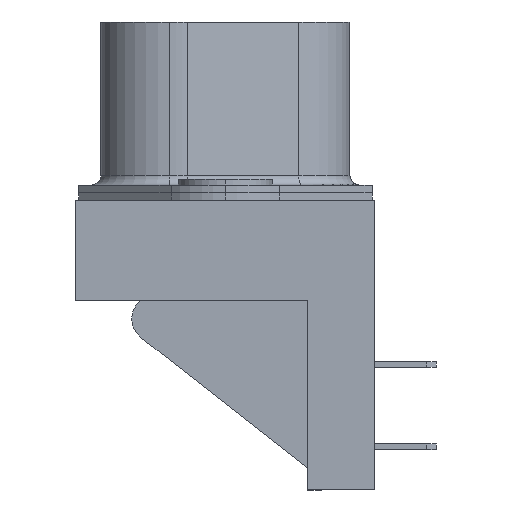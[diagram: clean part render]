
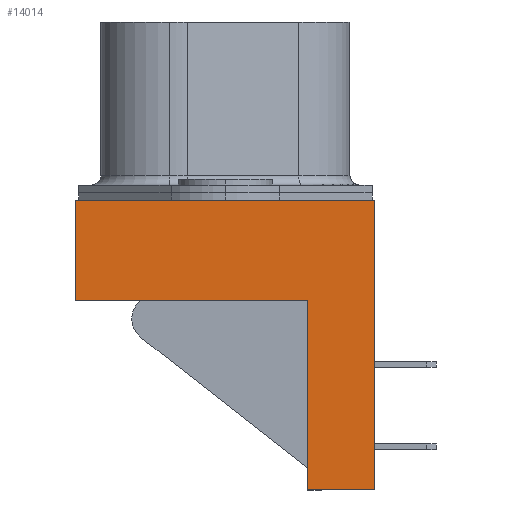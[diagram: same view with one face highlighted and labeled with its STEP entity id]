
A CAD part, left-side view. The second image highlights one B-rep face of the part: STEP entity #14014.
In plain terms, the highlighted planar face has unit normal (-1, 0, 0).
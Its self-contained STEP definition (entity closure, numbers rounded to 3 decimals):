
#9369 = VECTOR ( 'NONE', #12311, 1000. ) ;
#9684 = VECTOR ( 'NONE', #60644, 1000. ) ;
#11759 = AXIS2_PLACEMENT_3D ( 'NONE', #77047, #102448, #144937 ) ;
#12311 = DIRECTION ( 'NONE',  ( 0., 0., 1. ) ) ;
#14014 = ADVANCED_FACE ( 'NONE', ( #63472 ), #129609, .T. ) ;
#18101 = CARTESIAN_POINT ( 'NONE',  ( -4.125, 7.8, -5.2 ) ) ;
#22136 = DIRECTION ( 'NONE',  ( 0., -1., 0. ) ) ;
#24438 = VERTEX_POINT ( 'NONE', #119259 ) ;
#33593 = EDGE_CURVE ( 'NONE', #167851, #145563, #58864, .T. ) ;
#37057 = LINE ( 'NONE', #165261, #9369 ) ;
#38082 = LINE ( 'NONE', #151143, #132666 ) ;
#38355 = EDGE_CURVE ( 'NONE', #89803, #167851, #37057, .T. ) ;
#39267 = EDGE_LOOP ( 'NONE', ( #99872, #169555, #94851, #153107, #139628, #147882 ) ) ;
#40729 = DIRECTION ( 'NONE',  ( 0., 0., 1. ) ) ;
#41414 = LINE ( 'NONE', #83108, #78340 ) ;
#44869 = DIRECTION ( 'NONE',  ( 0., -1., 0. ) ) ;
#58864 = LINE ( 'NONE', #18101, #9684 ) ;
#60644 = DIRECTION ( 'NONE',  ( 0., 1., 0. ) ) ;
#63472 = FACE_OUTER_BOUND ( 'NONE', #39267, .T. ) ;
#72490 = EDGE_CURVE ( 'NONE', #145563, #24438, #38082, .T. ) ;
#75844 = EDGE_CURVE ( 'NONE', #24438, #79515, #104523, .T. ) ;
#77047 = CARTESIAN_POINT ( 'NONE',  ( -4.125, 7.8, -15.1 ) ) ;
#77162 = CARTESIAN_POINT ( 'NONE',  ( -4.125, -7.8, -15.1 ) ) ;
#78340 = VECTOR ( 'NONE', #99342, 1000. ) ;
#79515 = VERTEX_POINT ( 'NONE', #103573 ) ;
#83108 = CARTESIAN_POINT ( 'NONE',  ( -4.125, -7.8, -15.1 ) ) ;
#85628 = CARTESIAN_POINT ( 'NONE',  ( -4.125, 7.8, -15.1 ) ) ;
#89803 = VERTEX_POINT ( 'NONE', #178020 ) ;
#93838 = VECTOR ( 'NONE', #44869, 1000. ) ;
#94851 = ORIENTED_EDGE ( 'NONE', *, *, #155749, .T. ) ;
#99342 = DIRECTION ( 'NONE',  ( 0., 0., 1. ) ) ;
#99872 = ORIENTED_EDGE ( 'NONE', *, *, #33593, .F. ) ;
#102448 = DIRECTION ( 'NONE',  ( -1., 0., 0. ) ) ;
#103573 = CARTESIAN_POINT ( 'NONE',  ( -4.125, -7.8, 0. ) ) ;
#104523 = LINE ( 'NONE', #146140, #139546 ) ;
#111916 = EDGE_CURVE ( 'NONE', #177104, #79515, #41414, .T. ) ;
#117256 = CARTESIAN_POINT ( 'NONE',  ( -4.125, -4.3, -5.2 ) ) ;
#119259 = CARTESIAN_POINT ( 'NONE',  ( -4.125, 7.8, 0. ) ) ;
#129609 = PLANE ( 'NONE',  #11759 ) ;
#132666 = VECTOR ( 'NONE', #40729, 1000. ) ;
#139546 = VECTOR ( 'NONE', #22136, 1000. ) ;
#139628 = ORIENTED_EDGE ( 'NONE', *, *, #75844, .F. ) ;
#141716 = LINE ( 'NONE', #85628, #93838 ) ;
#144937 = DIRECTION ( 'NONE',  ( 0., -1., 0. ) ) ;
#145563 = VERTEX_POINT ( 'NONE', #159196 ) ;
#146140 = CARTESIAN_POINT ( 'NONE',  ( -4.125, 7.8, 0. ) ) ;
#147882 = ORIENTED_EDGE ( 'NONE', *, *, #72490, .F. ) ;
#151143 = CARTESIAN_POINT ( 'NONE',  ( -4.125, 7.8, -15.1 ) ) ;
#153107 = ORIENTED_EDGE ( 'NONE', *, *, #111916, .T. ) ;
#155749 = EDGE_CURVE ( 'NONE', #89803, #177104, #141716, .T. ) ;
#159196 = CARTESIAN_POINT ( 'NONE',  ( -4.125, 7.8, -5.2 ) ) ;
#165261 = CARTESIAN_POINT ( 'NONE',  ( -4.125, -4.3, -15.1 ) ) ;
#167851 = VERTEX_POINT ( 'NONE', #117256 ) ;
#169555 = ORIENTED_EDGE ( 'NONE', *, *, #38355, .F. ) ;
#177104 = VERTEX_POINT ( 'NONE', #77162 ) ;
#178020 = CARTESIAN_POINT ( 'NONE',  ( -4.125, -4.3, -15.1 ) ) ;
